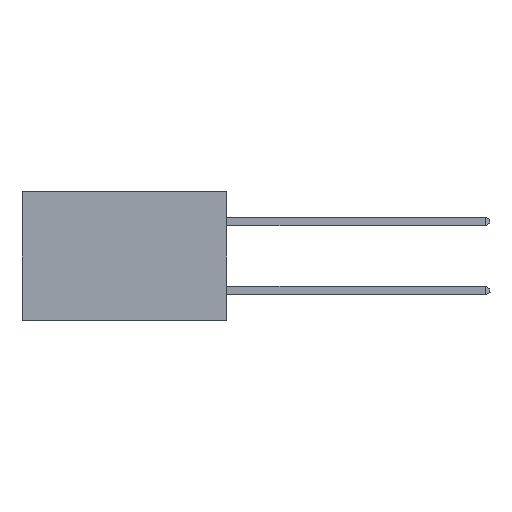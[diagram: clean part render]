
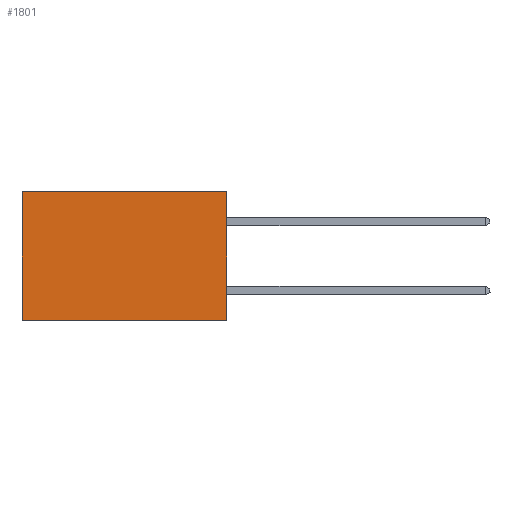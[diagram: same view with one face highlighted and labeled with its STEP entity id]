
A CAD part, left-side view. The second image highlights one B-rep face of the part: STEP entity #1801.
In plain terms, the highlighted planar face has unit normal (-1, 0, 0).
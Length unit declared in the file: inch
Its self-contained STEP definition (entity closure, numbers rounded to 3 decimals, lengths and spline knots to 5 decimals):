
#116 = DIRECTION ( 'NONE',  ( 0., 1., 0. ) ) ;
#252 = VECTOR ( 'NONE', #6240, 39.37008 ) ;
#638 = DIRECTION ( 'NONE',  ( 0., 1., 0. ) ) ;
#1017 = AXIS2_PLACEMENT_3D ( 'NONE', #16549, #3725, #12718 ) ;
#1207 = LINE ( 'NONE', #9093, #14503 ) ;
#1801 = ADVANCED_FACE ( 'NONE', ( #8377 ), #11449, .F. ) ;
#2528 = ORIENTED_EDGE ( 'NONE', *, *, #3233, .F. ) ;
#2807 = VECTOR ( 'NONE', #638, 39.37008 ) ;
#2813 = EDGE_CURVE ( 'NONE', #5930, #9901, #16594, .T. ) ;
#3153 = VERTEX_POINT ( 'NONE', #8633 ) ;
#3233 = EDGE_CURVE ( 'NONE', #3153, #4267, #16576, .T. ) ;
#3725 = DIRECTION ( 'NONE',  ( 1., 0., 0. ) ) ;
#4267 = VERTEX_POINT ( 'NONE', #10582 ) ;
#5930 = VERTEX_POINT ( 'NONE', #13127 ) ;
#6240 = DIRECTION ( 'NONE',  ( 0., 0., -1. ) ) ;
#6718 = VECTOR ( 'NONE', #11824, 39.37008 ) ;
#7536 = ORIENTED_EDGE ( 'NONE', *, *, #7854, .T. ) ;
#7653 = EDGE_LOOP ( 'NONE', ( #12472, #16147, #2528, #7536 ) ) ;
#7854 = EDGE_CURVE ( 'NONE', #3153, #5930, #1207, .T. ) ;
#8004 = CARTESIAN_POINT ( 'NONE',  ( 0.277, 0.59, -0.37 ) ) ;
#8210 = EDGE_CURVE ( 'NONE', #4267, #9901, #16498, .T. ) ;
#8377 = FACE_OUTER_BOUND ( 'NONE', #7653, .T. ) ;
#8633 = CARTESIAN_POINT ( 'NONE',  ( 0.277, 0., 0. ) ) ;
#8968 = CARTESIAN_POINT ( 'NONE',  ( 0.277, 0.59, -0.37 ) ) ;
#9093 = CARTESIAN_POINT ( 'NONE',  ( 0.277, 0., 0. ) ) ;
#9617 = CARTESIAN_POINT ( 'NONE',  ( 0.277, 0., -0.37 ) ) ;
#9901 = VERTEX_POINT ( 'NONE', #8968 ) ;
#10582 = CARTESIAN_POINT ( 'NONE',  ( 0.277, 0., -0.37 ) ) ;
#11449 = PLANE ( 'NONE',  #1017 ) ;
#11824 = DIRECTION ( 'NONE',  ( 0., 0., -1. ) ) ;
#12472 = ORIENTED_EDGE ( 'NONE', *, *, #2813, .T. ) ;
#12718 = DIRECTION ( 'NONE',  ( 0., 0., -1. ) ) ;
#13127 = CARTESIAN_POINT ( 'NONE',  ( 0.277, 0.59, 0. ) ) ;
#13966 = CARTESIAN_POINT ( 'NONE',  ( 0.277, 0., -0.37 ) ) ;
#14503 = VECTOR ( 'NONE', #116, 39.37008 ) ;
#16147 = ORIENTED_EDGE ( 'NONE', *, *, #8210, .F. ) ;
#16498 = LINE ( 'NONE', #9617, #2807 ) ;
#16549 = CARTESIAN_POINT ( 'NONE',  ( 0.277, 0., -0.37 ) ) ;
#16576 = LINE ( 'NONE', #13966, #252 ) ;
#16594 = LINE ( 'NONE', #8004, #6718 ) ;
